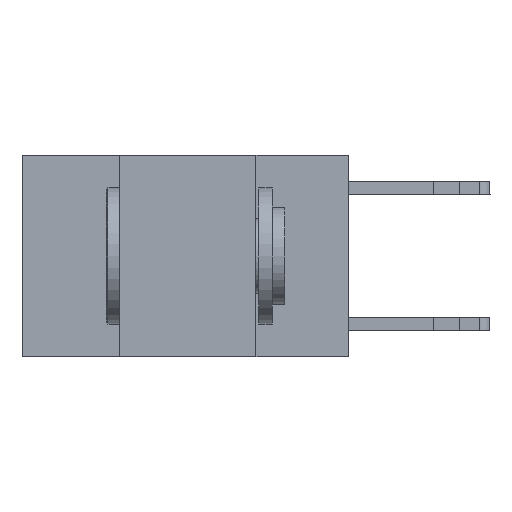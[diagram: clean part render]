
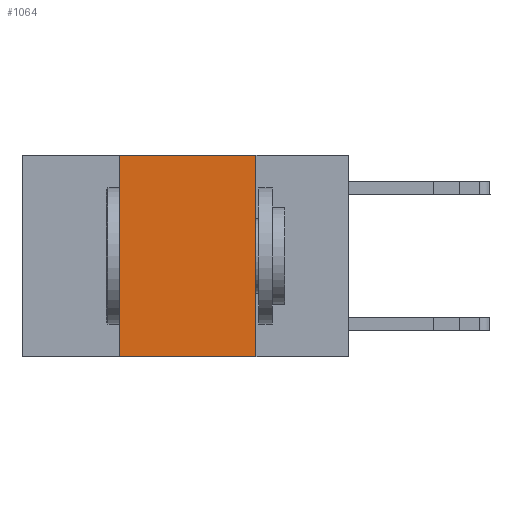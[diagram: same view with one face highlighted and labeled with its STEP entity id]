
A CAD part, left-side view. The second image highlights one B-rep face of the part: STEP entity #1064.
In plain terms, the highlighted planar face has unit normal (-1, 0, 0).
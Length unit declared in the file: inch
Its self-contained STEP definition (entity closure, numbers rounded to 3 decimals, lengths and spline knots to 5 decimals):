
#723 = DIRECTION ( 'NONE',  ( 0., -1., 0. ) ) ;
#894 = EDGE_CURVE ( 'NONE', #1957, #8328, #7904, .T. ) ;
#1064 = ADVANCED_FACE ( 'NONE', ( #1189 ), #9475, .F. ) ;
#1096 = DIRECTION ( 'NONE',  ( 1., 0., 0. ) ) ;
#1189 = FACE_OUTER_BOUND ( 'NONE', #16277, .T. ) ;
#1643 = LINE ( 'NONE', #8913, #3796 ) ;
#1957 = VERTEX_POINT ( 'NONE', #2515 ) ;
#2515 = CARTESIAN_POINT ( 'NONE',  ( 0., 0.42, -0.37 ) ) ;
#2905 = DIRECTION ( 'NONE',  ( 0., -1., 0. ) ) ;
#3796 = VECTOR ( 'NONE', #11751, 39.37008 ) ;
#4783 = CARTESIAN_POINT ( 'NONE',  ( 0., 0.42, 0. ) ) ;
#4868 = VECTOR ( 'NONE', #723, 39.37008 ) ;
#5137 = EDGE_CURVE ( 'NONE', #1957, #5819, #6776, .T. ) ;
#5331 = VECTOR ( 'NONE', #18010, 39.37008 ) ;
#5819 = VERTEX_POINT ( 'NONE', #13935 ) ;
#6179 = ORIENTED_EDGE ( 'NONE', *, *, #894, .T. ) ;
#6776 = LINE ( 'NONE', #4783, #5331 ) ;
#6936 = AXIS2_PLACEMENT_3D ( 'NONE', #13973, #1096, #17937 ) ;
#7193 = ORIENTED_EDGE ( 'NONE', *, *, #5137, .F. ) ;
#7904 = LINE ( 'NONE', #12029, #4868 ) ;
#8328 = VERTEX_POINT ( 'NONE', #16290 ) ;
#8913 = CARTESIAN_POINT ( 'NONE',  ( 0., 0.17, 0. ) ) ;
#9475 = PLANE ( 'NONE',  #6936 ) ;
#9888 = VECTOR ( 'NONE', #2905, 39.37008 ) ;
#10904 = LINE ( 'NONE', #14139, #9888 ) ;
#11751 = DIRECTION ( 'NONE',  ( 0., 0., -1. ) ) ;
#12029 = CARTESIAN_POINT ( 'NONE',  ( 0., 0.6, -0.37 ) ) ;
#12420 = EDGE_CURVE ( 'NONE', #16149, #8328, #1643, .T. ) ;
#13180 = ORIENTED_EDGE ( 'NONE', *, *, #12420, .F. ) ;
#13935 = CARTESIAN_POINT ( 'NONE',  ( 0., 0.42, 0. ) ) ;
#13973 = CARTESIAN_POINT ( 'NONE',  ( 0., 0.6, 0. ) ) ;
#14139 = CARTESIAN_POINT ( 'NONE',  ( 0., 0.6, 0. ) ) ;
#14890 = EDGE_CURVE ( 'NONE', #5819, #16149, #10904, .T. ) ;
#16061 = ORIENTED_EDGE ( 'NONE', *, *, #14890, .F. ) ;
#16149 = VERTEX_POINT ( 'NONE', #17930 ) ;
#16277 = EDGE_LOOP ( 'NONE', ( #13180, #16061, #7193, #6179 ) ) ;
#16290 = CARTESIAN_POINT ( 'NONE',  ( 0., 0.17, -0.37 ) ) ;
#17930 = CARTESIAN_POINT ( 'NONE',  ( 0., 0.17, 0. ) ) ;
#17937 = DIRECTION ( 'NONE',  ( 0., 0., -1. ) ) ;
#18010 = DIRECTION ( 'NONE',  ( 0., 0., 1. ) ) ;
